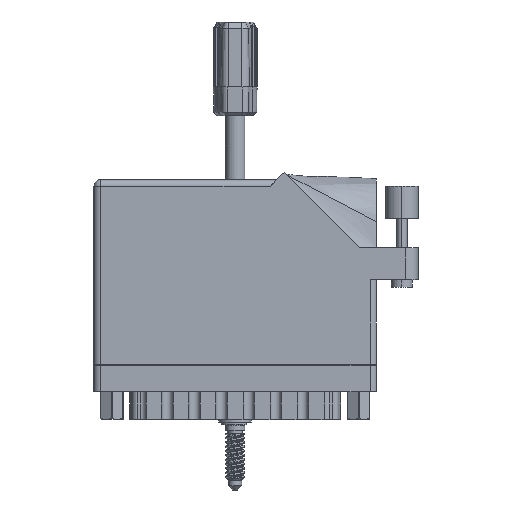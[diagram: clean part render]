
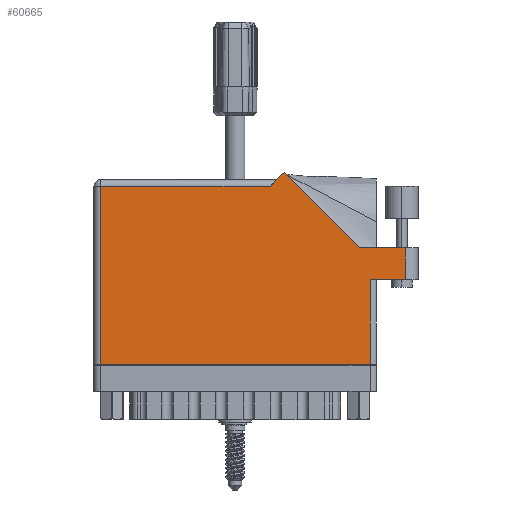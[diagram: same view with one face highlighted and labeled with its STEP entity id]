
A CAD part, front view. The second image highlights one B-rep face of the part: STEP entity #60665.
In plain terms, the highlighted face is planar.
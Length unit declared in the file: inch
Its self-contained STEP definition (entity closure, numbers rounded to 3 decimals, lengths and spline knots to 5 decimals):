
#2636 = LINE ( 'NONE', #32968, #68136 ) ;
#4489 = CARTESIAN_POINT ( 'NONE',  ( 0.062, 1.713, 0. ) ) ;
#6599 = LINE ( 'NONE', #18035, #39244 ) ;
#8153 = EDGE_CURVE ( 'NONE', #33943, #14004, #79958, .T. ) ;
#9697 = CARTESIAN_POINT ( 'NONE',  ( 2.55242, 1.122, 0. ) ) ;
#9722 = ORIENTED_EDGE ( 'NONE', *, *, #8153, .T. ) ;
#13698 = DIRECTION ( 'NONE',  ( -1., 0., 0. ) ) ;
#14004 = VERTEX_POINT ( 'NONE', #53087 ) ;
#14797 = LINE ( 'NONE', #64189, #68903 ) ;
#14888 = VERTEX_POINT ( 'NONE', #25825 ) ;
#15949 = VERTEX_POINT ( 'NONE', #4489 ) ;
#17686 = DIRECTION ( 'NONE',  ( -0.707, -0.707, 0. ) ) ;
#17988 = CARTESIAN_POINT ( 'NONE',  ( 1.758, 1.775, 0. ) ) ;
#18035 = CARTESIAN_POINT ( 'NONE',  ( 0., 0., 0. ) ) ;
#18240 = LINE ( 'NONE', #17988, #73528 ) ;
#19180 = CARTESIAN_POINT ( 'NONE',  ( 0.062, 0., 0. ) ) ;
#20763 = CARTESIAN_POINT ( 'NONE',  ( 0., 1.713, 0. ) ) ;
#21338 = CARTESIAN_POINT ( 'NONE',  ( 2.993, 0.815, 0. ) ) ;
#21560 = DIRECTION ( 'NONE',  ( -1., 0., 0. ) ) ;
#22552 = ORIENTED_EDGE ( 'NONE', *, *, #34283, .T. ) ;
#25587 = ORIENTED_EDGE ( 'NONE', *, *, #26287, .T. ) ;
#25825 = CARTESIAN_POINT ( 'NONE',  ( 1.696, 1.713, 0. ) ) ;
#26287 = EDGE_CURVE ( 'NONE', #14004, #53143, #2636, .T. ) ;
#27533 = FACE_OUTER_BOUND ( 'NONE', #38224, .T. ) ;
#31613 = DIRECTION ( 'NONE',  ( 0., 1., 0. ) ) ;
#32968 = CARTESIAN_POINT ( 'NONE',  ( 2.718, 0.815, 0. ) ) ;
#33657 = VECTOR ( 'NONE', #76246, 39.37008 ) ;
#33943 = VERTEX_POINT ( 'NONE', #80544 ) ;
#34283 = EDGE_CURVE ( 'NONE', #52962, #14888, #18240, .T. ) ;
#35147 = ORIENTED_EDGE ( 'NONE', *, *, #52282, .T. ) ;
#36046 = VECTOR ( 'NONE', #47820, 39.37008 ) ;
#36183 = VERTEX_POINT ( 'NONE', #9697 ) ;
#37187 = CARTESIAN_POINT ( 'NONE',  ( 2.993, 1.122, 0. ) ) ;
#38224 = EDGE_LOOP ( 'NONE', ( #25587, #67368, #79330, #43775, #22552, #43213, #52612, #35147, #9722 ) ) ;
#39244 = VECTOR ( 'NONE', #75415, 39.37008 ) ;
#40721 = EDGE_CURVE ( 'NONE', #36183, #52962, #57513, .T. ) ;
#43213 = ORIENTED_EDGE ( 'NONE', *, *, #71398, .T. ) ;
#43775 = ORIENTED_EDGE ( 'NONE', *, *, #40721, .T. ) ;
#47820 = DIRECTION ( 'NONE',  ( -0.707, 0.707, 0. ) ) ;
#48473 = VERTEX_POINT ( 'NONE', #64719 ) ;
#49664 = CARTESIAN_POINT ( 'NONE',  ( 0., 1.775, 0. ) ) ;
#52282 = EDGE_CURVE ( 'NONE', #48473, #33943, #6599, .T. ) ;
#52612 = ORIENTED_EDGE ( 'NONE', *, *, #66082, .T. ) ;
#52868 = LINE ( 'NONE', #19180, #33657 ) ;
#52962 = VERTEX_POINT ( 'NONE', #75616 ) ;
#53087 = CARTESIAN_POINT ( 'NONE',  ( 2.656, 0.815, 0. ) ) ;
#53143 = VERTEX_POINT ( 'NONE', #21338 ) ;
#54258 = VECTOR ( 'NONE', #92949, 39.37008 ) ;
#54769 = CARTESIAN_POINT ( 'NONE',  ( 2.55242, 1.122, 0. ) ) ;
#57180 = AXIS2_PLACEMENT_3D ( 'NONE', #49664, #57516, #13698 ) ;
#57513 = LINE ( 'NONE', #54769, #36046 ) ;
#57516 = DIRECTION ( 'NONE',  ( 0., 0., -1. ) ) ;
#58025 = VECTOR ( 'NONE', #31613, 39.37008 ) ;
#60665 = ADVANCED_FACE ( 'NONE', ( #27533 ), #79221, .F. ) ;
#60791 = VECTOR ( 'NONE', #65177, 39.37008 ) ;
#61387 = DIRECTION ( 'NONE',  ( 1., 0., 0. ) ) ;
#62558 = LINE ( 'NONE', #74864, #58025 ) ;
#62838 = EDGE_CURVE ( 'NONE', #90236, #36183, #14797, .T. ) ;
#64189 = CARTESIAN_POINT ( 'NONE',  ( 3.118, 1.122, 0. ) ) ;
#64719 = CARTESIAN_POINT ( 'NONE',  ( 0.062, 0., 0. ) ) ;
#65177 = DIRECTION ( 'NONE',  ( 0., 1., 0. ) ) ;
#66082 = EDGE_CURVE ( 'NONE', #15949, #48473, #52868, .T. ) ;
#67368 = ORIENTED_EDGE ( 'NONE', *, *, #78152, .T. ) ;
#68136 = VECTOR ( 'NONE', #61387, 39.37008 ) ;
#68903 = VECTOR ( 'NONE', #21560, 39.37008 ) ;
#71158 = CARTESIAN_POINT ( 'NONE',  ( 2.656, 0.815, 0. ) ) ;
#71398 = EDGE_CURVE ( 'NONE', #14888, #15949, #92599, .T. ) ;
#73528 = VECTOR ( 'NONE', #17686, 39.37008 ) ;
#74864 = CARTESIAN_POINT ( 'NONE',  ( 2.993, 1.122, 0. ) ) ;
#75415 = DIRECTION ( 'NONE',  ( 1., 0., 0. ) ) ;
#75616 = CARTESIAN_POINT ( 'NONE',  ( 1.82871, 1.84571, 0. ) ) ;
#76246 = DIRECTION ( 'NONE',  ( 0., -1., 0. ) ) ;
#78152 = EDGE_CURVE ( 'NONE', #53143, #90236, #62558, .T. ) ;
#79221 = PLANE ( 'NONE',  #57180 ) ;
#79330 = ORIENTED_EDGE ( 'NONE', *, *, #62838, .T. ) ;
#79958 = LINE ( 'NONE', #71158, #60791 ) ;
#80544 = CARTESIAN_POINT ( 'NONE',  ( 2.656, 0., 0. ) ) ;
#90236 = VERTEX_POINT ( 'NONE', #37187 ) ;
#92599 = LINE ( 'NONE', #20763, #54258 ) ;
#92949 = DIRECTION ( 'NONE',  ( -1., 0., 0. ) ) ;
